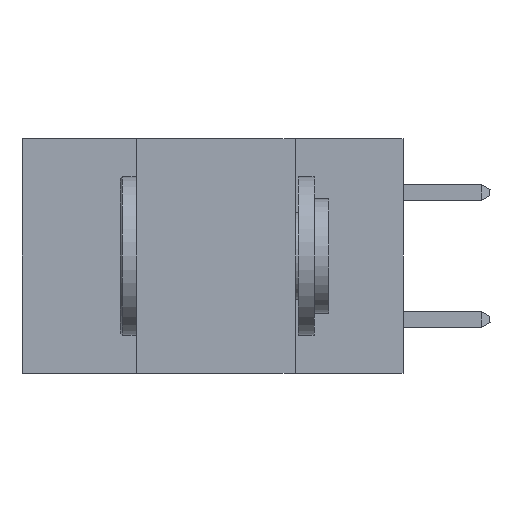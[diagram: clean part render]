
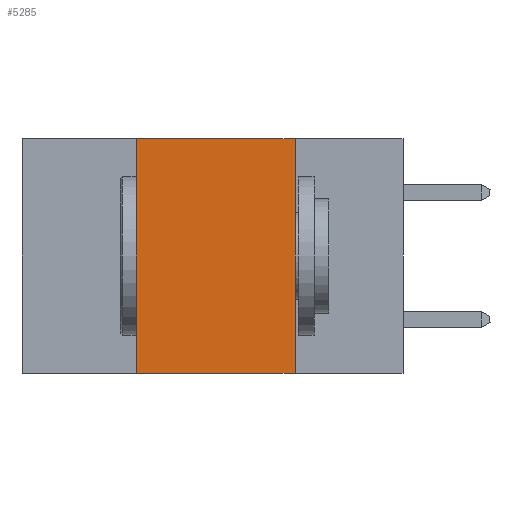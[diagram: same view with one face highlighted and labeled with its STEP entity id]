
A CAD part, left-side view. The second image highlights one B-rep face of the part: STEP entity #5285.
In plain terms, the highlighted planar face has unit normal (-1, 0, 0).
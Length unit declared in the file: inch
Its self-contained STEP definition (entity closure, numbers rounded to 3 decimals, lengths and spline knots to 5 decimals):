
#47 = CARTESIAN_POINT ( 'NONE',  ( 0., 0.17, 0. ) ) ;
#443 = LINE ( 'NONE', #9799, #7174 ) ;
#1205 = VERTEX_POINT ( 'NONE', #8105 ) ;
#1338 = CARTESIAN_POINT ( 'NONE',  ( 0., 0.6, 0. ) ) ;
#3108 = VECTOR ( 'NONE', #11855, 39.37008 ) ;
#3662 = VECTOR ( 'NONE', #9310, 39.37008 ) ;
#3748 = EDGE_LOOP ( 'NONE', ( #4438, #4030, #6648, #11132 ) ) ;
#4030 = ORIENTED_EDGE ( 'NONE', *, *, #6225, .F. ) ;
#4438 = ORIENTED_EDGE ( 'NONE', *, *, #13230, .F. ) ;
#4489 = LINE ( 'NONE', #47, #14393 ) ;
#5285 = ADVANCED_FACE ( 'NONE', ( #13673 ), #11059, .F. ) ;
#6225 = EDGE_CURVE ( 'NONE', #10309, #1205, #13645, .T. ) ;
#6648 = ORIENTED_EDGE ( 'NONE', *, *, #15987, .F. ) ;
#7174 = VECTOR ( 'NONE', #11087, 39.37008 ) ;
#7519 = CARTESIAN_POINT ( 'NONE',  ( 0., 0.42, -0.37 ) ) ;
#7845 = CARTESIAN_POINT ( 'NONE',  ( 0., 0.42, 0. ) ) ;
#8105 = CARTESIAN_POINT ( 'NONE',  ( 0., 0.17, 0. ) ) ;
#9310 = DIRECTION ( 'NONE',  ( 0., -1., 0. ) ) ;
#9384 = DIRECTION ( 'NONE',  ( 0., 0., -1. ) ) ;
#9458 = VERTEX_POINT ( 'NONE', #11380 ) ;
#9799 = CARTESIAN_POINT ( 'NONE',  ( 0., 0.42, 0. ) ) ;
#10143 = LINE ( 'NONE', #10548, #3108 ) ;
#10309 = VERTEX_POINT ( 'NONE', #7845 ) ;
#10386 = EDGE_CURVE ( 'NONE', #12920, #9458, #10143, .T. ) ;
#10548 = CARTESIAN_POINT ( 'NONE',  ( 0., 0.6, -0.37 ) ) ;
#10624 = DIRECTION ( 'NONE',  ( 0., 0., -1. ) ) ;
#10643 = DIRECTION ( 'NONE',  ( 1., 0., 0. ) ) ;
#10738 = CARTESIAN_POINT ( 'NONE',  ( 0., 0.6, 0. ) ) ;
#11059 = PLANE ( 'NONE',  #11217 ) ;
#11087 = DIRECTION ( 'NONE',  ( 0., 0., 1. ) ) ;
#11132 = ORIENTED_EDGE ( 'NONE', *, *, #10386, .T. ) ;
#11217 = AXIS2_PLACEMENT_3D ( 'NONE', #10738, #10643, #10624 ) ;
#11380 = CARTESIAN_POINT ( 'NONE',  ( 0., 0.17, -0.37 ) ) ;
#11855 = DIRECTION ( 'NONE',  ( 0., -1., 0. ) ) ;
#12920 = VERTEX_POINT ( 'NONE', #7519 ) ;
#13230 = EDGE_CURVE ( 'NONE', #1205, #9458, #4489, .T. ) ;
#13645 = LINE ( 'NONE', #1338, #3662 ) ;
#13673 = FACE_OUTER_BOUND ( 'NONE', #3748, .T. ) ;
#14393 = VECTOR ( 'NONE', #9384, 39.37008 ) ;
#15987 = EDGE_CURVE ( 'NONE', #12920, #10309, #443, .T. ) ;
